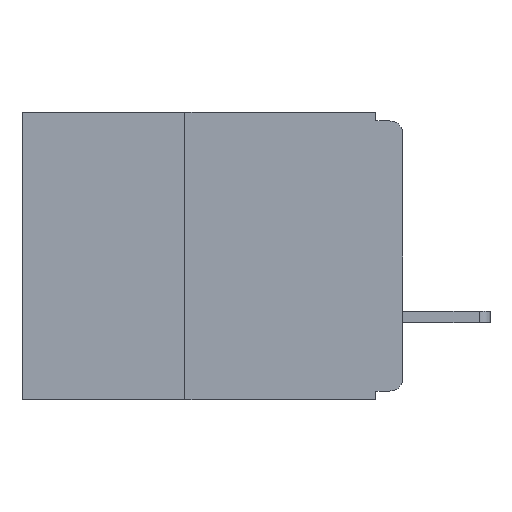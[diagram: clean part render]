
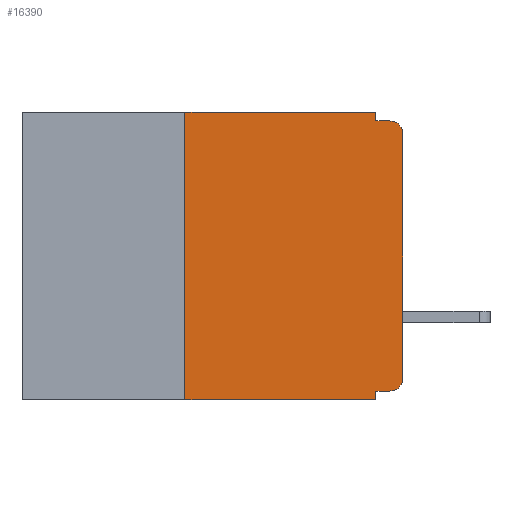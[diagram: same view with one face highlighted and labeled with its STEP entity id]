
A CAD part, left-side view. The second image highlights one B-rep face of the part: STEP entity #16390.
In plain terms, the highlighted planar face has unit normal (-1, 0, 0).
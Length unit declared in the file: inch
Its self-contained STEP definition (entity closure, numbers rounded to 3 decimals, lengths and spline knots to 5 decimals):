
#12 = EDGE_CURVE ( 'NONE', #3346, #32524, #12907, .T. ) ;
#554 = EDGE_CURVE ( 'NONE', #29198, #1678, #22722, .T. ) ;
#575 = CARTESIAN_POINT ( 'NONE',  ( 0., 0.25, -0.33 ) ) ;
#673 = CARTESIAN_POINT ( 'NONE',  ( 0., 0.015, -0.01 ) ) ;
#844 = EDGE_CURVE ( 'NONE', #22013, #31970, #2240, .T. ) ;
#1153 = LINE ( 'NONE', #2390, #8136 ) ;
#1198 = ORIENTED_EDGE ( 'NONE', *, *, #8892, .T. ) ;
#1678 = VERTEX_POINT ( 'NONE', #8835 ) ;
#1860 = VECTOR ( 'NONE', #5524, 39.37008 ) ;
#1922 = DIRECTION ( 'NONE',  ( 0., 1., 0. ) ) ;
#1984 = LINE ( 'NONE', #17846, #8945 ) ;
#2088 = DIRECTION ( 'NONE',  ( -1., 0., 0. ) ) ;
#2190 = DIRECTION ( 'NONE',  ( 0., 0., -1. ) ) ;
#2240 = LINE ( 'NONE', #3653, #18159 ) ;
#2390 = CARTESIAN_POINT ( 'NONE',  ( 0., 0.437, -0.33 ) ) ;
#3009 = CARTESIAN_POINT ( 'NONE',  ( 0., 0.031, 0. ) ) ;
#3159 = VECTOR ( 'NONE', #28337, 39.37008 ) ;
#3346 = VERTEX_POINT ( 'NONE', #16044 ) ;
#3653 = CARTESIAN_POINT ( 'NONE',  ( 0., 0.031, -0.33 ) ) ;
#3982 = DIRECTION ( 'NONE',  ( -1., 0., 0. ) ) ;
#4553 = AXIS2_PLACEMENT_3D ( 'NONE', #17740, #2088, #20381 ) ;
#5165 = EDGE_CURVE ( 'NONE', #30810, #11806, #31408, .T. ) ;
#5265 = EDGE_CURVE ( 'NONE', #11806, #32524, #14997, .T. ) ;
#5524 = DIRECTION ( 'NONE',  ( 0., 0., 1. ) ) ;
#6004 = VECTOR ( 'NONE', #12465, 39.37008 ) ;
#6076 = CARTESIAN_POINT ( 'NONE',  ( 0., 0., 0. ) ) ;
#6523 = CARTESIAN_POINT ( 'NONE',  ( 0., 0.437, 0. ) ) ;
#7550 = DIRECTION ( 'NONE',  ( 0., -1., 0. ) ) ;
#7851 = ORIENTED_EDGE ( 'NONE', *, *, #554, .F. ) ;
#8029 = VERTEX_POINT ( 'NONE', #24110 ) ;
#8136 = VECTOR ( 'NONE', #7550, 39.37008 ) ;
#8825 = ORIENTED_EDGE ( 'NONE', *, *, #33376, .F. ) ;
#8835 = CARTESIAN_POINT ( 'NONE',  ( 0., 0.25, 0. ) ) ;
#8892 = EDGE_CURVE ( 'NONE', #8029, #30810, #24916, .T. ) ;
#8945 = VECTOR ( 'NONE', #2190, 39.37008 ) ;
#11635 = VERTEX_POINT ( 'NONE', #3009 ) ;
#11684 = ORIENTED_EDGE ( 'NONE', *, *, #12, .F. ) ;
#11806 = VERTEX_POINT ( 'NONE', #21981 ) ;
#12411 = CARTESIAN_POINT ( 'NONE',  ( 0., 0., -0.32 ) ) ;
#12465 = DIRECTION ( 'NONE',  ( 0., -1., 0. ) ) ;
#12907 = LINE ( 'NONE', #31062, #6004 ) ;
#14149 = VECTOR ( 'NONE', #1922, 39.37008 ) ;
#14251 = EDGE_LOOP ( 'NONE', ( #16814, #14435, #11684, #8825, #29113, #7851, #33513, #22567, #26980, #1198 ) ) ;
#14435 = ORIENTED_EDGE ( 'NONE', *, *, #5265, .T. ) ;
#14997 = CIRCLE ( 'NONE', #21806, 0.015 ) ;
#16044 = CARTESIAN_POINT ( 'NONE',  ( 0., 0.031, -0.01 ) ) ;
#16390 = ADVANCED_FACE ( 'NONE', ( #17304 ), #27468, .F. ) ;
#16814 = ORIENTED_EDGE ( 'NONE', *, *, #5165, .T. ) ;
#17027 = DIRECTION ( 'NONE',  ( 0., 0., -1. ) ) ;
#17304 = FACE_OUTER_BOUND ( 'NONE', #14251, .T. ) ;
#17479 = VECTOR ( 'NONE', #29629, 39.37008 ) ;
#17740 = CARTESIAN_POINT ( 'NONE',  ( 0., 0.015, -0.305 ) ) ;
#17846 = CARTESIAN_POINT ( 'NONE',  ( 0., 0.031, 0. ) ) ;
#18159 = VECTOR ( 'NONE', #27848, 39.37008 ) ;
#19656 = CARTESIAN_POINT ( 'NONE',  ( 0., 0.015, -0.025 ) ) ;
#20381 = DIRECTION ( 'NONE',  ( 0., 0., -1. ) ) ;
#21195 = EDGE_CURVE ( 'NONE', #29198, #31970, #1153, .T. ) ;
#21801 = EDGE_CURVE ( 'NONE', #1678, #11635, #30191, .T. ) ;
#21806 = AXIS2_PLACEMENT_3D ( 'NONE', #19656, #3982, #22283 ) ;
#21903 = CARTESIAN_POINT ( 'NONE',  ( 0., 0.031, -0.32 ) ) ;
#21981 = CARTESIAN_POINT ( 'NONE',  ( 0., 0., -0.025 ) ) ;
#22013 = VERTEX_POINT ( 'NONE', #21903 ) ;
#22283 = DIRECTION ( 'NONE',  ( 0., 0., -1. ) ) ;
#22567 = ORIENTED_EDGE ( 'NONE', *, *, #844, .F. ) ;
#22722 = LINE ( 'NONE', #575, #1860 ) ;
#24110 = CARTESIAN_POINT ( 'NONE',  ( 0., 0.015, -0.32 ) ) ;
#24524 = CARTESIAN_POINT ( 'NONE',  ( 0., 0.25, -0.33 ) ) ;
#24779 = EDGE_CURVE ( 'NONE', #8029, #22013, #28109, .T. ) ;
#24916 = CIRCLE ( 'NONE', #4553, 0.015 ) ;
#26318 = AXIS2_PLACEMENT_3D ( 'NONE', #6523, #32699, #17027 ) ;
#26980 = ORIENTED_EDGE ( 'NONE', *, *, #24779, .F. ) ;
#27119 = CARTESIAN_POINT ( 'NONE',  ( 0., 0., -0.305 ) ) ;
#27468 = PLANE ( 'NONE',  #26318 ) ;
#27848 = DIRECTION ( 'NONE',  ( 0., 0., -1. ) ) ;
#28109 = LINE ( 'NONE', #12411, #14149 ) ;
#28337 = DIRECTION ( 'NONE',  ( 0., -1., 0. ) ) ;
#29113 = ORIENTED_EDGE ( 'NONE', *, *, #21801, .F. ) ;
#29198 = VERTEX_POINT ( 'NONE', #24524 ) ;
#29629 = DIRECTION ( 'NONE',  ( 0., 0., 1. ) ) ;
#30191 = LINE ( 'NONE', #33590, #3159 ) ;
#30810 = VERTEX_POINT ( 'NONE', #27119 ) ;
#31062 = CARTESIAN_POINT ( 'NONE',  ( 0., 0., -0.01 ) ) ;
#31408 = LINE ( 'NONE', #6076, #17479 ) ;
#31970 = VERTEX_POINT ( 'NONE', #32513 ) ;
#32513 = CARTESIAN_POINT ( 'NONE',  ( 0., 0.031, -0.33 ) ) ;
#32524 = VERTEX_POINT ( 'NONE', #673 ) ;
#32699 = DIRECTION ( 'NONE',  ( 1., 0., 0. ) ) ;
#33376 = EDGE_CURVE ( 'NONE', #11635, #3346, #1984, .T. ) ;
#33513 = ORIENTED_EDGE ( 'NONE', *, *, #21195, .T. ) ;
#33590 = CARTESIAN_POINT ( 'NONE',  ( 0., 0.437, 0. ) ) ;
